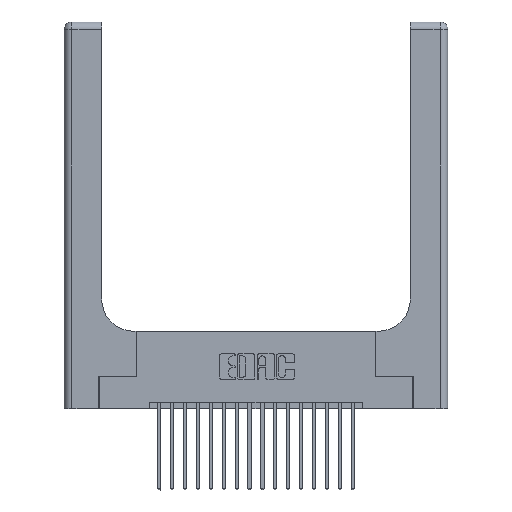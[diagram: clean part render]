
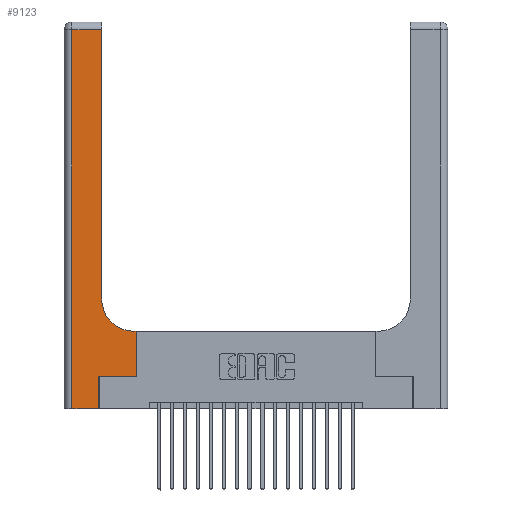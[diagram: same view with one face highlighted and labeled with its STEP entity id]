
A CAD part, top view. The second image highlights one B-rep face of the part: STEP entity #9123.
In plain terms, the highlighted planar face has unit normal (0, 0, 1).
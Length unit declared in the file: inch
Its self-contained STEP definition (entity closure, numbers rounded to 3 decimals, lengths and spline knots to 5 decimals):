
#246 = CARTESIAN_POINT ( 'NONE',  ( 0., 0., 0.37 ) ) ;
#430 = DIRECTION ( 'NONE',  ( 0., 1., 0. ) ) ;
#472 = CARTESIAN_POINT ( 'NONE',  ( 0., 2.94, 0.37 ) ) ;
#669 = EDGE_CURVE ( 'NONE', #18911, #2692, #2282, .T. ) ;
#742 = CARTESIAN_POINT ( 'NONE',  ( 0.5585, 0.6, 0.37 ) ) ;
#943 = CARTESIAN_POINT ( 'NONE',  ( 0.2915, 3., 0.37 ) ) ;
#1085 = ORIENTED_EDGE ( 'NONE', *, *, #7360, .T. ) ;
#1095 = VECTOR ( 'NONE', #4696, 39.37008 ) ;
#1216 = CARTESIAN_POINT ( 'NONE',  ( 0.06, 2.94, 0.37 ) ) ;
#1350 = VECTOR ( 'NONE', #430, 39.37008 ) ;
#1546 = CARTESIAN_POINT ( 'NONE',  ( 0.2915, 2.94, 0.37 ) ) ;
#1936 = AXIS2_PLACEMENT_3D ( 'NONE', #11756, #18414, #2276 ) ;
#2045 = ORIENTED_EDGE ( 'NONE', *, *, #669, .T. ) ;
#2068 = PLANE ( 'NONE',  #1936 ) ;
#2276 = DIRECTION ( 'NONE',  ( -1., 0., 0. ) ) ;
#2278 = VECTOR ( 'NONE', #18650, 39.37008 ) ;
#2282 = LINE ( 'NONE', #246, #10484 ) ;
#2453 = CIRCLE ( 'NONE', #18127, 0.25 ) ;
#2692 = VERTEX_POINT ( 'NONE', #11026 ) ;
#3157 = CARTESIAN_POINT ( 'NONE',  ( 0.5415, 0.85, 0.37 ) ) ;
#3772 = EDGE_CURVE ( 'NONE', #10927, #15274, #15921, .T. ) ;
#4014 = LINE ( 'NONE', #20106, #6590 ) ;
#4696 = DIRECTION ( 'NONE',  ( 1., 0., 0. ) ) ;
#4877 = EDGE_CURVE ( 'NONE', #12980, #8737, #19242, .T. ) ;
#5292 = ORIENTED_EDGE ( 'NONE', *, *, #3772, .T. ) ;
#5545 = CARTESIAN_POINT ( 'NONE',  ( 0.2915, 0.6, 0.37 ) ) ;
#5730 = LINE ( 'NONE', #20177, #15725 ) ;
#6590 = VECTOR ( 'NONE', #15473, 39.37008 ) ;
#6942 = EDGE_CURVE ( 'NONE', #8737, #10927, #2453, .T. ) ;
#7360 = EDGE_CURVE ( 'NONE', #2692, #13861, #4014, .T. ) ;
#8134 = DIRECTION ( 'NONE',  ( 0., 0., -1. ) ) ;
#8737 = VERTEX_POINT ( 'NONE', #15487 ) ;
#9080 = FACE_OUTER_BOUND ( 'NONE', #13537, .T. ) ;
#9123 = ADVANCED_FACE ( 'NONE', ( #9080 ), #2068, .F. ) ;
#9352 = EDGE_CURVE ( 'NONE', #13420, #12980, #17777, .T. ) ;
#9575 = LINE ( 'NONE', #19381, #1095 ) ;
#9577 = CARTESIAN_POINT ( 'NONE',  ( 0.2915, 0.85, 0.37 ) ) ;
#9687 = VECTOR ( 'NONE', #20350, 39.37008 ) ;
#10224 = CARTESIAN_POINT ( 'NONE',  ( 0.06, 0., 0.37 ) ) ;
#10257 = DIRECTION ( 'NONE',  ( 1., 0., 0. ) ) ;
#10391 = DIRECTION ( 'NONE',  ( 0., -1., 0. ) ) ;
#10484 = VECTOR ( 'NONE', #10257, 39.37008 ) ;
#10927 = VERTEX_POINT ( 'NONE', #9577 ) ;
#11026 = CARTESIAN_POINT ( 'NONE',  ( 0.269, 0., 0.37 ) ) ;
#11756 = CARTESIAN_POINT ( 'NONE',  ( 0., 3., 0.37 ) ) ;
#11799 = ORIENTED_EDGE ( 'NONE', *, *, #15889, .T. ) ;
#11895 = ORIENTED_EDGE ( 'NONE', *, *, #6942, .T. ) ;
#12375 = EDGE_CURVE ( 'NONE', #15274, #17660, #14029, .T. ) ;
#12948 = CARTESIAN_POINT ( 'NONE',  ( 0.269, 0.25, 0.37 ) ) ;
#12980 = VERTEX_POINT ( 'NONE', #742 ) ;
#13420 = VERTEX_POINT ( 'NONE', #16356 ) ;
#13537 = EDGE_LOOP ( 'NONE', ( #5292, #16772, #19588, #2045, #1085, #11799, #18047, #17085, #11895 ) ) ;
#13861 = VERTEX_POINT ( 'NONE', #12948 ) ;
#14029 = LINE ( 'NONE', #472, #9687 ) ;
#15274 = VERTEX_POINT ( 'NONE', #1546 ) ;
#15466 = EDGE_CURVE ( 'NONE', #17660, #18911, #5730, .T. ) ;
#15473 = DIRECTION ( 'NONE',  ( 0., 1., 0. ) ) ;
#15487 = CARTESIAN_POINT ( 'NONE',  ( 0.5415, 0.6, 0.37 ) ) ;
#15725 = VECTOR ( 'NONE', #10391, 39.37008 ) ;
#15889 = EDGE_CURVE ( 'NONE', #13861, #13420, #9575, .T. ) ;
#15921 = LINE ( 'NONE', #943, #17211 ) ;
#16356 = CARTESIAN_POINT ( 'NONE',  ( 0.5585, 0.25, 0.37 ) ) ;
#16758 = CARTESIAN_POINT ( 'NONE',  ( 0.5585, 0.25, 0.37 ) ) ;
#16772 = ORIENTED_EDGE ( 'NONE', *, *, #12375, .T. ) ;
#17085 = ORIENTED_EDGE ( 'NONE', *, *, #4877, .T. ) ;
#17211 = VECTOR ( 'NONE', #20614, 39.37008 ) ;
#17660 = VERTEX_POINT ( 'NONE', #1216 ) ;
#17777 = LINE ( 'NONE', #16758, #1350 ) ;
#18047 = ORIENTED_EDGE ( 'NONE', *, *, #9352, .T. ) ;
#18127 = AXIS2_PLACEMENT_3D ( 'NONE', #3157, #8134, #19570 ) ;
#18414 = DIRECTION ( 'NONE',  ( 0., 0., -1. ) ) ;
#18650 = DIRECTION ( 'NONE',  ( -1., 0., 0. ) ) ;
#18911 = VERTEX_POINT ( 'NONE', #10224 ) ;
#19242 = LINE ( 'NONE', #5545, #2278 ) ;
#19381 = CARTESIAN_POINT ( 'NONE',  ( 0.269, 0.25, 0.37 ) ) ;
#19570 = DIRECTION ( 'NONE',  ( 1., 0., 0. ) ) ;
#19588 = ORIENTED_EDGE ( 'NONE', *, *, #15466, .T. ) ;
#20106 = CARTESIAN_POINT ( 'NONE',  ( 0.269, 0., 0.37 ) ) ;
#20177 = CARTESIAN_POINT ( 'NONE',  ( 0.06, 3., 0.37 ) ) ;
#20350 = DIRECTION ( 'NONE',  ( -1., 0., 0. ) ) ;
#20614 = DIRECTION ( 'NONE',  ( 0., 1., 0. ) ) ;
